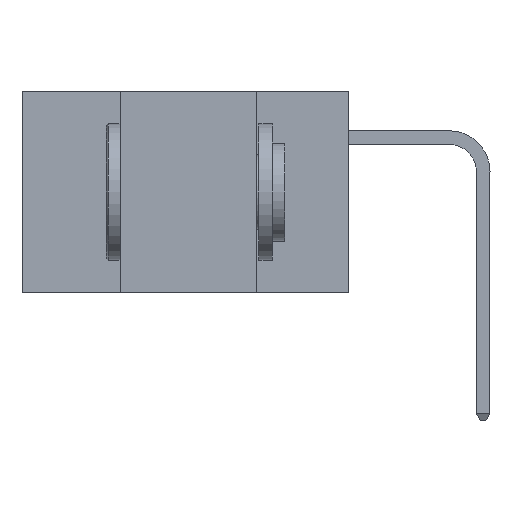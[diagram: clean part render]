
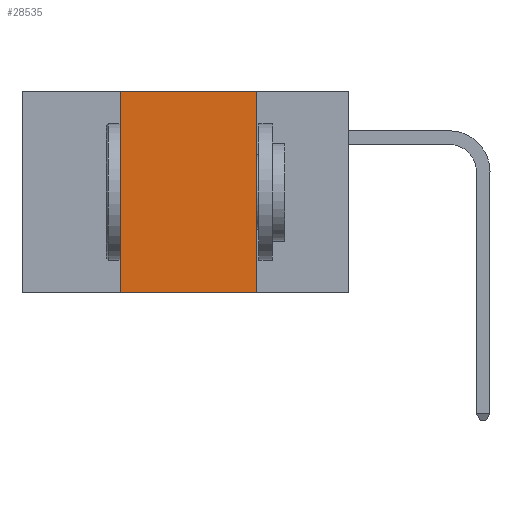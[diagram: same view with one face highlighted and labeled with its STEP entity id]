
A CAD part, left-side view. The second image highlights one B-rep face of the part: STEP entity #28535.
In plain terms, the highlighted planar face has unit normal (-1, 0, 0).
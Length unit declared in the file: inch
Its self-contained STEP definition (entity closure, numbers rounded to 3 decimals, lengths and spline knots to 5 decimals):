
#357 = VERTEX_POINT ( 'NONE', #19922 ) ;
#661 = LINE ( 'NONE', #27122, #31186 ) ;
#3365 = ORIENTED_EDGE ( 'NONE', *, *, #16257, .F. ) ;
#4190 = EDGE_CURVE ( 'NONE', #17863, #357, #23733, .T. ) ;
#4809 = EDGE_CURVE ( 'NONE', #10300, #357, #661, .T. ) ;
#5199 = CARTESIAN_POINT ( 'NONE',  ( 0., 0.17, 0. ) ) ;
#5200 = VERTEX_POINT ( 'NONE', #23729 ) ;
#5556 = DIRECTION ( 'NONE',  ( 0., -1., 0. ) ) ;
#5658 = ORIENTED_EDGE ( 'NONE', *, *, #4809, .T. ) ;
#6142 = CARTESIAN_POINT ( 'NONE',  ( 0., 0.42, -0.37 ) ) ;
#8164 = DIRECTION ( 'NONE',  ( 0., 0., -1. ) ) ;
#9709 = DIRECTION ( 'NONE',  ( 0., 0., 1. ) ) ;
#10300 = VERTEX_POINT ( 'NONE', #6142 ) ;
#10340 = FACE_OUTER_BOUND ( 'NONE', #11981, .T. ) ;
#11967 = DIRECTION ( 'NONE',  ( 1., 0., 0. ) ) ;
#11981 = EDGE_LOOP ( 'NONE', ( #28215, #3365, #23332, #5658 ) ) ;
#13365 = LINE ( 'NONE', #18714, #25319 ) ;
#13819 = EDGE_CURVE ( 'NONE', #10300, #5200, #15749, .T. ) ;
#15749 = LINE ( 'NONE', #26478, #28442 ) ;
#15753 = AXIS2_PLACEMENT_3D ( 'NONE', #23885, #11967, #28700 ) ;
#16257 = EDGE_CURVE ( 'NONE', #5200, #17863, #13365, .T. ) ;
#16327 = DIRECTION ( 'NONE',  ( 0., -1., 0. ) ) ;
#17433 = VECTOR ( 'NONE', #8164, 39.37008 ) ;
#17863 = VERTEX_POINT ( 'NONE', #5199 ) ;
#18714 = CARTESIAN_POINT ( 'NONE',  ( 0., 0.6, 0. ) ) ;
#19922 = CARTESIAN_POINT ( 'NONE',  ( 0., 0.17, -0.37 ) ) ;
#21478 = PLANE ( 'NONE',  #15753 ) ;
#23332 = ORIENTED_EDGE ( 'NONE', *, *, #13819, .F. ) ;
#23729 = CARTESIAN_POINT ( 'NONE',  ( 0., 0.42, 0. ) ) ;
#23733 = LINE ( 'NONE', #29764, #17433 ) ;
#23885 = CARTESIAN_POINT ( 'NONE',  ( 0., 0.6, 0. ) ) ;
#25319 = VECTOR ( 'NONE', #16327, 39.37008 ) ;
#26478 = CARTESIAN_POINT ( 'NONE',  ( 0., 0.42, 0. ) ) ;
#27122 = CARTESIAN_POINT ( 'NONE',  ( 0., 0.6, -0.37 ) ) ;
#28215 = ORIENTED_EDGE ( 'NONE', *, *, #4190, .F. ) ;
#28442 = VECTOR ( 'NONE', #9709, 39.37008 ) ;
#28535 = ADVANCED_FACE ( 'NONE', ( #10340 ), #21478, .F. ) ;
#28700 = DIRECTION ( 'NONE',  ( 0., 0., -1. ) ) ;
#29764 = CARTESIAN_POINT ( 'NONE',  ( 0., 0.17, 0. ) ) ;
#31186 = VECTOR ( 'NONE', #5556, 39.37008 ) ;
